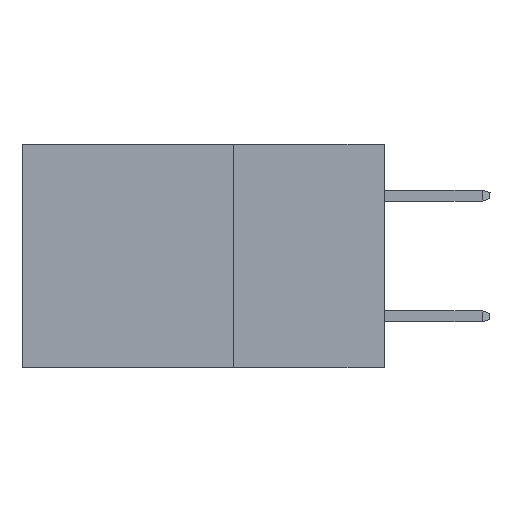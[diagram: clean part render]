
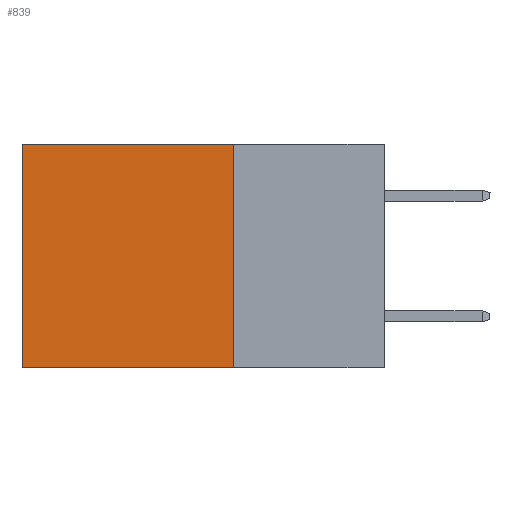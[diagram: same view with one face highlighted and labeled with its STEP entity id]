
A CAD part, left-side view. The second image highlights one B-rep face of the part: STEP entity #839.
In plain terms, the highlighted planar face has unit normal (-1, 0, 0).
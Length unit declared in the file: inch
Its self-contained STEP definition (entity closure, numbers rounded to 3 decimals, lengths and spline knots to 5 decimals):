
#455 = ORIENTED_EDGE ( 'NONE', *, *, #22899, .F. ) ;
#839 = ADVANCED_FACE ( 'NONE', ( #19703 ), #12892, .F. ) ;
#1646 = DIRECTION ( 'NONE',  ( 0., 0., -1. ) ) ;
#1688 = LINE ( 'NONE', #14678, #10239 ) ;
#3892 = EDGE_CURVE ( 'NONE', #9637, #4471, #1688, .T. ) ;
#3921 = EDGE_CURVE ( 'NONE', #20458, #11565, #7020, .T. ) ;
#4471 = VERTEX_POINT ( 'NONE', #13313 ) ;
#4622 = VECTOR ( 'NONE', #20168, 39.37008 ) ;
#4905 = AXIS2_PLACEMENT_3D ( 'NONE', #18347, #24020, #12808 ) ;
#4913 = DIRECTION ( 'NONE',  ( 0., 1., 0. ) ) ;
#5135 = CARTESIAN_POINT ( 'NONE',  ( 0.298, 0.25, 0. ) ) ;
#5606 = CARTESIAN_POINT ( 'NONE',  ( 0.298, 0.6, 0. ) ) ;
#6556 = VECTOR ( 'NONE', #4913, 39.37008 ) ;
#7015 = LINE ( 'NONE', #5135, #4622 ) ;
#7020 = LINE ( 'NONE', #18352, #20988 ) ;
#8435 = ORIENTED_EDGE ( 'NONE', *, *, #3921, .F. ) ;
#8618 = CARTESIAN_POINT ( 'NONE',  ( 0.298, 0.25, -0.37 ) ) ;
#9637 = VERTEX_POINT ( 'NONE', #5606 ) ;
#10239 = VECTOR ( 'NONE', #1646, 39.37008 ) ;
#10668 = LINE ( 'NONE', #8618, #6556 ) ;
#11565 = VERTEX_POINT ( 'NONE', #18461 ) ;
#12808 = DIRECTION ( 'NONE',  ( 0., 0., -1. ) ) ;
#12892 = PLANE ( 'NONE',  #4905 ) ;
#13313 = CARTESIAN_POINT ( 'NONE',  ( 0.298, 0.6, -0.37 ) ) ;
#14428 = DIRECTION ( 'NONE',  ( 0., 0., -1. ) ) ;
#14678 = CARTESIAN_POINT ( 'NONE',  ( 0.298, 0.6, 0. ) ) ;
#14762 = CARTESIAN_POINT ( 'NONE',  ( 0.298, 0.25, 0. ) ) ;
#14822 = ORIENTED_EDGE ( 'NONE', *, *, #19137, .T. ) ;
#14937 = EDGE_LOOP ( 'NONE', ( #20244, #455, #8435, #14822 ) ) ;
#18347 = CARTESIAN_POINT ( 'NONE',  ( 0.298, 0.25, 0. ) ) ;
#18352 = CARTESIAN_POINT ( 'NONE',  ( 0.298, 0.25, 0. ) ) ;
#18461 = CARTESIAN_POINT ( 'NONE',  ( 0.298, 0.25, -0.37 ) ) ;
#19137 = EDGE_CURVE ( 'NONE', #20458, #9637, #7015, .T. ) ;
#19703 = FACE_OUTER_BOUND ( 'NONE', #14937, .T. ) ;
#20168 = DIRECTION ( 'NONE',  ( 0., 1., 0. ) ) ;
#20244 = ORIENTED_EDGE ( 'NONE', *, *, #3892, .T. ) ;
#20458 = VERTEX_POINT ( 'NONE', #14762 ) ;
#20988 = VECTOR ( 'NONE', #14428, 39.37008 ) ;
#22899 = EDGE_CURVE ( 'NONE', #11565, #4471, #10668, .T. ) ;
#24020 = DIRECTION ( 'NONE',  ( 1., 0., 0. ) ) ;
